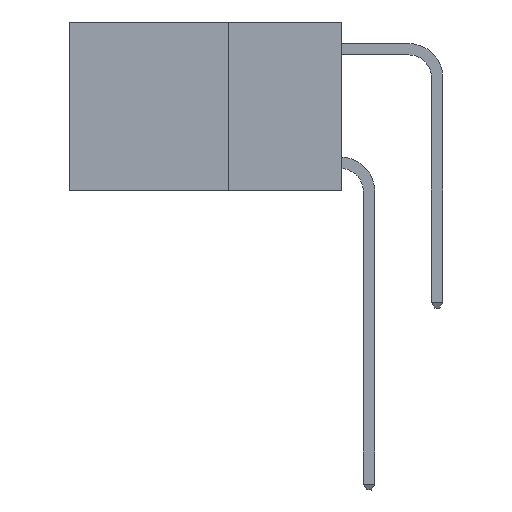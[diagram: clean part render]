
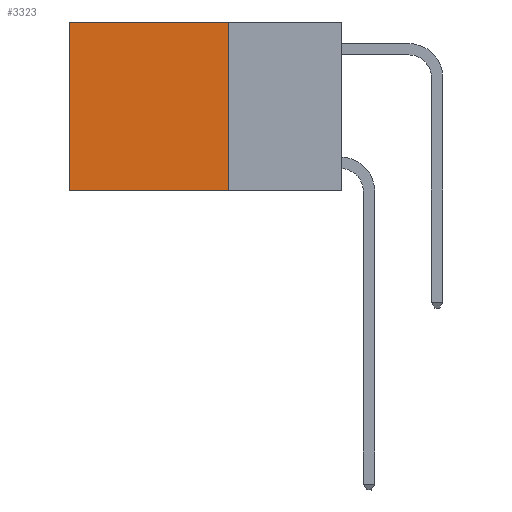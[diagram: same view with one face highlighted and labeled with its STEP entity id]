
A CAD part, left-side view. The second image highlights one B-rep face of the part: STEP entity #3323.
In plain terms, the highlighted planar face has unit normal (-1, 0, 0).
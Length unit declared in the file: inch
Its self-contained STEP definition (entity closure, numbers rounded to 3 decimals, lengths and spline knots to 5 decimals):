
#808 = DIRECTION ( 'NONE',  ( 0., 0., -1. ) ) ;
#1093 = ORIENTED_EDGE ( 'NONE', *, *, #28292, .F. ) ;
#1345 = DIRECTION ( 'NONE',  ( 0., 1., 0. ) ) ;
#1963 = ORIENTED_EDGE ( 'NONE', *, *, #30226, .F. ) ;
#3323 = ADVANCED_FACE ( 'NONE', ( #6445 ), #11519, .F. ) ;
#3595 = ORIENTED_EDGE ( 'NONE', *, *, #10584, .T. ) ;
#5530 = CARTESIAN_POINT ( 'NONE',  ( 0.2625, 0.6, 0. ) ) ;
#5604 = VECTOR ( 'NONE', #26217, 39.37008 ) ;
#6115 = VERTEX_POINT ( 'NONE', #31694 ) ;
#6445 = FACE_OUTER_BOUND ( 'NONE', #8498, .T. ) ;
#8162 = CARTESIAN_POINT ( 'NONE',  ( 0.2625, 0.25, -0.37 ) ) ;
#8498 = EDGE_LOOP ( 'NONE', ( #3595, #1093, #1963, #11020 ) ) ;
#8891 = VECTOR ( 'NONE', #808, 39.37008 ) ;
#10584 = EDGE_CURVE ( 'NONE', #13034, #6115, #23414, .T. ) ;
#11020 = ORIENTED_EDGE ( 'NONE', *, *, #26069, .T. ) ;
#11407 = CARTESIAN_POINT ( 'NONE',  ( 0.2625, 0.25, 0. ) ) ;
#11519 = PLANE ( 'NONE',  #26713 ) ;
#13034 = VERTEX_POINT ( 'NONE', #17243 ) ;
#13546 = DIRECTION ( 'NONE',  ( 1., 0., 0. ) ) ;
#13598 = LINE ( 'NONE', #11407, #8891 ) ;
#14129 = VECTOR ( 'NONE', #1345, 39.37008 ) ;
#16851 = CARTESIAN_POINT ( 'NONE',  ( 0.2625, 0.25, -0.37 ) ) ;
#17243 = CARTESIAN_POINT ( 'NONE',  ( 0.2625, 0.6, 0. ) ) ;
#21832 = CARTESIAN_POINT ( 'NONE',  ( 0.2625, 0.25, 0. ) ) ;
#23251 = DIRECTION ( 'NONE',  ( 0., 0., -1. ) ) ;
#23414 = LINE ( 'NONE', #5530, #25211 ) ;
#24949 = LINE ( 'NONE', #32350, #14129 ) ;
#25211 = VECTOR ( 'NONE', #23251, 39.37008 ) ;
#25490 = CARTESIAN_POINT ( 'NONE',  ( 0.2625, 0.25, 0. ) ) ;
#26069 = EDGE_CURVE ( 'NONE', #31448, #13034, #24949, .T. ) ;
#26217 = DIRECTION ( 'NONE',  ( 0., 1., 0. ) ) ;
#26713 = AXIS2_PLACEMENT_3D ( 'NONE', #21832, #13546, #32089 ) ;
#28292 = EDGE_CURVE ( 'NONE', #29828, #6115, #31096, .T. ) ;
#29828 = VERTEX_POINT ( 'NONE', #16851 ) ;
#30226 = EDGE_CURVE ( 'NONE', #31448, #29828, #13598, .T. ) ;
#31096 = LINE ( 'NONE', #8162, #5604 ) ;
#31448 = VERTEX_POINT ( 'NONE', #25490 ) ;
#31694 = CARTESIAN_POINT ( 'NONE',  ( 0.2625, 0.6, -0.37 ) ) ;
#32089 = DIRECTION ( 'NONE',  ( 0., 0., -1. ) ) ;
#32350 = CARTESIAN_POINT ( 'NONE',  ( 0.2625, 0.25, 0. ) ) ;
